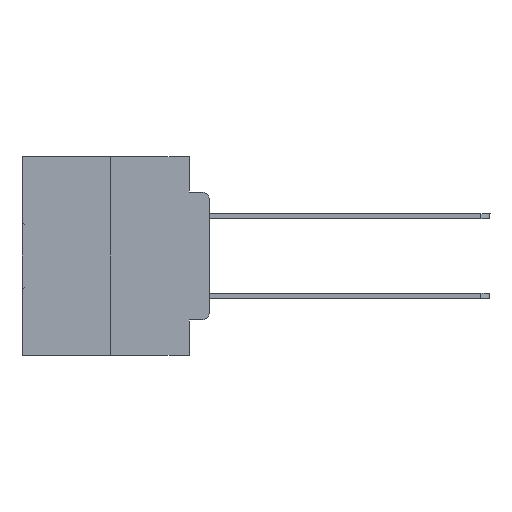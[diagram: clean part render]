
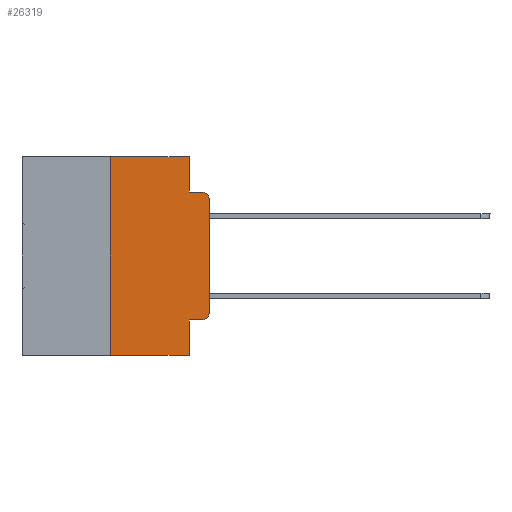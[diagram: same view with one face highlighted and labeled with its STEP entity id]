
A CAD part, left-side view. The second image highlights one B-rep face of the part: STEP entity #26319.
In plain terms, the highlighted planar face has unit normal (-1, 0, 0).
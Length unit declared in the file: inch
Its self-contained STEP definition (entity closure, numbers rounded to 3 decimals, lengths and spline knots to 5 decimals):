
#733 = LINE ( 'NONE', #21859, #9167 ) ;
#840 = DIRECTION ( 'NONE',  ( 0., -1., 0. ) ) ;
#1147 = DIRECTION ( 'NONE',  ( 0., 0., -1. ) ) ;
#1258 = EDGE_CURVE ( 'NONE', #3791, #19400, #20006, .T. ) ;
#1266 = VECTOR ( 'NONE', #2399, 39.37008 ) ;
#1340 = EDGE_CURVE ( 'NONE', #13888, #15479, #18060, .T. ) ;
#1384 = EDGE_CURVE ( 'NONE', #15479, #19422, #26048, .T. ) ;
#2235 = LINE ( 'NONE', #32103, #1266 ) ;
#2399 = DIRECTION ( 'NONE',  ( 0., -1., 0. ) ) ;
#2460 = EDGE_CURVE ( 'NONE', #5411, #19422, #8412, .T. ) ;
#2725 = ORIENTED_EDGE ( 'NONE', *, *, #15741, .F. ) ;
#3791 = VERTEX_POINT ( 'NONE', #5635 ) ;
#3921 = VECTOR ( 'NONE', #1147, 39.37008 ) ;
#4175 = AXIS2_PLACEMENT_3D ( 'NONE', #29132, #12581, #26151 ) ;
#4338 = CARTESIAN_POINT ( 'NONE',  ( 0., 0., -0.1085 ) ) ;
#5411 = VERTEX_POINT ( 'NONE', #20410 ) ;
#5635 = CARTESIAN_POINT ( 'NONE',  ( 0., 0.25, 0. ) ) ;
#6005 = EDGE_CURVE ( 'NONE', #29614, #16093, #2235, .T. ) ;
#7499 = DIRECTION ( 'NONE',  ( 0., 0., 1. ) ) ;
#7516 = DIRECTION ( 'NONE',  ( 0., -1., 0. ) ) ;
#7704 = CARTESIAN_POINT ( 'NONE',  ( 0., 0.051, -0.4115 ) ) ;
#8412 = LINE ( 'NONE', #34291, #12882 ) ;
#8938 = ORIENTED_EDGE ( 'NONE', *, *, #22132, .T. ) ;
#8981 = DIRECTION ( 'NONE',  ( 1., 0., 0. ) ) ;
#9167 = VECTOR ( 'NONE', #11444, 39.37008 ) ;
#10513 = AXIS2_PLACEMENT_3D ( 'NONE', #19717, #8981, #15278 ) ;
#11299 = CARTESIAN_POINT ( 'NONE',  ( 0., 0.25, -0.5 ) ) ;
#11444 = DIRECTION ( 'NONE',  ( 0., 0., 1. ) ) ;
#11615 = CARTESIAN_POINT ( 'NONE',  ( 0., 0.02, -0.4115 ) ) ;
#12042 = ORIENTED_EDGE ( 'NONE', *, *, #19210, .F. ) ;
#12581 = DIRECTION ( 'NONE',  ( -1., 0., 0. ) ) ;
#12882 = VECTOR ( 'NONE', #20967, 39.37008 ) ;
#13644 = VECTOR ( 'NONE', #840, 39.37008 ) ;
#13888 = VERTEX_POINT ( 'NONE', #29850 ) ;
#13975 = CARTESIAN_POINT ( 'NONE',  ( 0., 0.051, 0. ) ) ;
#14182 = CARTESIAN_POINT ( 'NONE',  ( 0., 0.473, 0. ) ) ;
#14938 = CARTESIAN_POINT ( 'NONE',  ( 0., 0.051, 0. ) ) ;
#15278 = DIRECTION ( 'NONE',  ( 0., 0., -1. ) ) ;
#15453 = DIRECTION ( 'NONE',  ( -1., 0., 0. ) ) ;
#15479 = VERTEX_POINT ( 'NONE', #4338 ) ;
#15741 = EDGE_CURVE ( 'NONE', #29614, #18707, #27009, .T. ) ;
#16093 = VERTEX_POINT ( 'NONE', #11615 ) ;
#16465 = EDGE_LOOP ( 'NONE', ( #17969, #29800, #23879, #30195, #27240, #12042, #8938, #2725, #30399, #25999 ) ) ;
#17018 = CIRCLE ( 'NONE', #21534, 0.02 ) ;
#17581 = VECTOR ( 'NONE', #7499, 39.37008 ) ;
#17969 = ORIENTED_EDGE ( 'NONE', *, *, #1340, .T. ) ;
#18060 = LINE ( 'NONE', #25977, #17581 ) ;
#18707 = VERTEX_POINT ( 'NONE', #24173 ) ;
#18791 = VECTOR ( 'NONE', #7516, 39.37008 ) ;
#18983 = VECTOR ( 'NONE', #29987, 39.37008 ) ;
#19210 = EDGE_CURVE ( 'NONE', #32051, #3791, #733, .T. ) ;
#19259 = LINE ( 'NONE', #13975, #3921 ) ;
#19400 = VERTEX_POINT ( 'NONE', #14938 ) ;
#19422 = VERTEX_POINT ( 'NONE', #30446 ) ;
#19524 = EDGE_CURVE ( 'NONE', #16093, #13888, #17018, .T. ) ;
#19611 = CARTESIAN_POINT ( 'NONE',  ( 0., 0.051, 0. ) ) ;
#19717 = CARTESIAN_POINT ( 'NONE',  ( 0., 0.473, 0. ) ) ;
#20006 = LINE ( 'NONE', #14182, #13644 ) ;
#20410 = CARTESIAN_POINT ( 'NONE',  ( 0., 0.051, -0.0885 ) ) ;
#20898 = LINE ( 'NONE', #31613, #18791 ) ;
#20967 = DIRECTION ( 'NONE',  ( 0., -1., 0. ) ) ;
#21534 = AXIS2_PLACEMENT_3D ( 'NONE', #26384, #15453, #26037 ) ;
#21859 = CARTESIAN_POINT ( 'NONE',  ( 0., 0.25, 0. ) ) ;
#22132 = EDGE_CURVE ( 'NONE', #32051, #18707, #20898, .T. ) ;
#23879 = ORIENTED_EDGE ( 'NONE', *, *, #2460, .F. ) ;
#24173 = CARTESIAN_POINT ( 'NONE',  ( 0., 0.051, -0.5 ) ) ;
#24997 = FACE_OUTER_BOUND ( 'NONE', #16465, .T. ) ;
#25977 = CARTESIAN_POINT ( 'NONE',  ( 0., 0., 0. ) ) ;
#25999 = ORIENTED_EDGE ( 'NONE', *, *, #19524, .T. ) ;
#26037 = DIRECTION ( 'NONE',  ( 0., 0., -1. ) ) ;
#26048 = CIRCLE ( 'NONE', #4175, 0.02 ) ;
#26151 = DIRECTION ( 'NONE',  ( 0., 0., -1. ) ) ;
#26319 = ADVANCED_FACE ( 'NONE', ( #24997 ), #33072, .F. ) ;
#26384 = CARTESIAN_POINT ( 'NONE',  ( 0., 0.02, -0.3915 ) ) ;
#27009 = LINE ( 'NONE', #19611, #18983 ) ;
#27240 = ORIENTED_EDGE ( 'NONE', *, *, #1258, .F. ) ;
#29042 = EDGE_CURVE ( 'NONE', #19400, #5411, #19259, .T. ) ;
#29132 = CARTESIAN_POINT ( 'NONE',  ( 0., 0.02, -0.1085 ) ) ;
#29614 = VERTEX_POINT ( 'NONE', #7704 ) ;
#29800 = ORIENTED_EDGE ( 'NONE', *, *, #1384, .T. ) ;
#29850 = CARTESIAN_POINT ( 'NONE',  ( 0., 0., -0.3915 ) ) ;
#29987 = DIRECTION ( 'NONE',  ( 0., 0., -1. ) ) ;
#30195 = ORIENTED_EDGE ( 'NONE', *, *, #29042, .F. ) ;
#30399 = ORIENTED_EDGE ( 'NONE', *, *, #6005, .T. ) ;
#30446 = CARTESIAN_POINT ( 'NONE',  ( 0., 0.02, -0.0885 ) ) ;
#31613 = CARTESIAN_POINT ( 'NONE',  ( 0., 0.473, -0.5 ) ) ;
#32051 = VERTEX_POINT ( 'NONE', #11299 ) ;
#32103 = CARTESIAN_POINT ( 'NONE',  ( 0., 0.051, -0.4115 ) ) ;
#33072 = PLANE ( 'NONE',  #10513 ) ;
#34291 = CARTESIAN_POINT ( 'NONE',  ( 0., 0.051, -0.0885 ) ) ;
